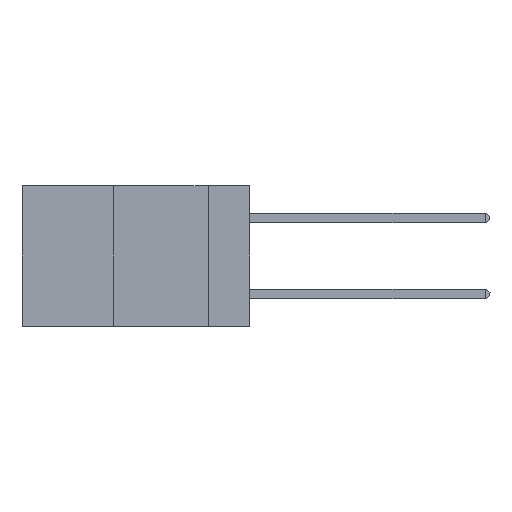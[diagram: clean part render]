
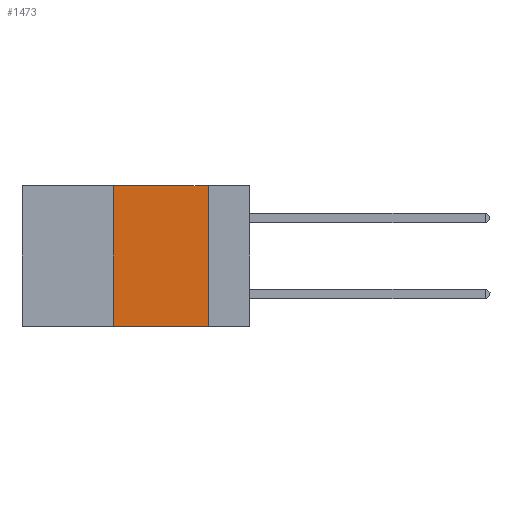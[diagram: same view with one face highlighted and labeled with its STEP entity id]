
A CAD part, left-side view. The second image highlights one B-rep face of the part: STEP entity #1473.
In plain terms, the highlighted planar face has unit normal (-1, 0, 0).
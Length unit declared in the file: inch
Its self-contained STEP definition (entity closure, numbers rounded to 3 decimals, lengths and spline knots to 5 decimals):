
#105 = CARTESIAN_POINT ( 'NONE',  ( 0., 0.11, 0. ) ) ;
#290 = LINE ( 'NONE', #4462, #8416 ) ;
#378 = DIRECTION ( 'NONE',  ( 0., -1., 0. ) ) ;
#382 = LINE ( 'NONE', #2804, #6370 ) ;
#721 = LINE ( 'NONE', #5955, #5449 ) ;
#1473 = ADVANCED_FACE ( 'NONE', ( #9708 ), #2666, .F. ) ;
#1540 = ORIENTED_EDGE ( 'NONE', *, *, #6885, .F. ) ;
#1867 = EDGE_LOOP ( 'NONE', ( #8505, #5052, #1540, #3675 ) ) ;
#2076 = LINE ( 'NONE', #105, #8206 ) ;
#2666 = PLANE ( 'NONE',  #3952 ) ;
#2804 = CARTESIAN_POINT ( 'NONE',  ( 0., 0.6, -0.37 ) ) ;
#3675 = ORIENTED_EDGE ( 'NONE', *, *, #8458, .T. ) ;
#3952 = AXIS2_PLACEMENT_3D ( 'NONE', #9695, #5828, #9057 ) ;
#4462 = CARTESIAN_POINT ( 'NONE',  ( 0., 0.36, 0. ) ) ;
#4861 = DIRECTION ( 'NONE',  ( 0., 0., -1. ) ) ;
#5052 = ORIENTED_EDGE ( 'NONE', *, *, #7213, .F. ) ;
#5274 = CARTESIAN_POINT ( 'NONE',  ( 0., 0.36, 0. ) ) ;
#5449 = VECTOR ( 'NONE', #7544, 39.37008 ) ;
#5538 = CARTESIAN_POINT ( 'NONE',  ( 0., 0.11, 0. ) ) ;
#5828 = DIRECTION ( 'NONE',  ( 1., 0., 0. ) ) ;
#5955 = CARTESIAN_POINT ( 'NONE',  ( 0., 0.6, 0. ) ) ;
#6249 = DIRECTION ( 'NONE',  ( 0., 0., 1. ) ) ;
#6337 = CARTESIAN_POINT ( 'NONE',  ( 0., 0.36, -0.37 ) ) ;
#6370 = VECTOR ( 'NONE', #378, 39.37008 ) ;
#6396 = VERTEX_POINT ( 'NONE', #5538 ) ;
#6885 = EDGE_CURVE ( 'NONE', #8096, #7918, #290, .T. ) ;
#7213 = EDGE_CURVE ( 'NONE', #7918, #6396, #721, .T. ) ;
#7544 = DIRECTION ( 'NONE',  ( 0., -1., 0. ) ) ;
#7712 = EDGE_CURVE ( 'NONE', #6396, #9219, #2076, .T. ) ;
#7816 = CARTESIAN_POINT ( 'NONE',  ( 0., 0.11, -0.37 ) ) ;
#7918 = VERTEX_POINT ( 'NONE', #5274 ) ;
#8096 = VERTEX_POINT ( 'NONE', #6337 ) ;
#8206 = VECTOR ( 'NONE', #4861, 39.37008 ) ;
#8416 = VECTOR ( 'NONE', #6249, 39.37008 ) ;
#8458 = EDGE_CURVE ( 'NONE', #8096, #9219, #382, .T. ) ;
#8505 = ORIENTED_EDGE ( 'NONE', *, *, #7712, .F. ) ;
#9057 = DIRECTION ( 'NONE',  ( 0., 0., -1. ) ) ;
#9219 = VERTEX_POINT ( 'NONE', #7816 ) ;
#9695 = CARTESIAN_POINT ( 'NONE',  ( 0., 0.6, 0. ) ) ;
#9708 = FACE_OUTER_BOUND ( 'NONE', #1867, .T. ) ;
